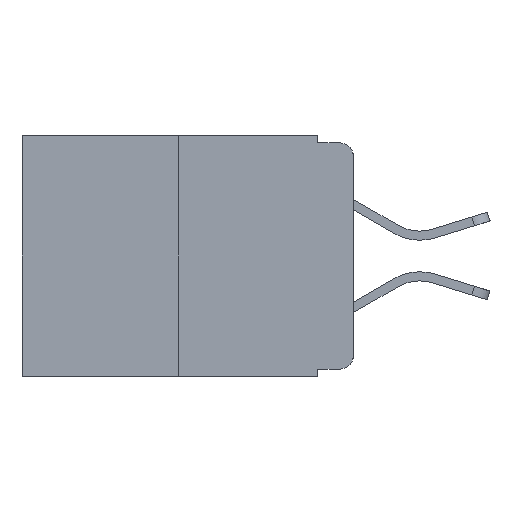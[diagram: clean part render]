
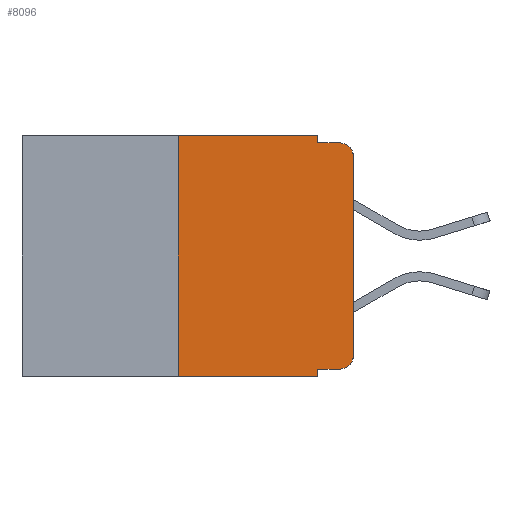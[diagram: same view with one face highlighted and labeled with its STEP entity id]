
A CAD part, left-side view. The second image highlights one B-rep face of the part: STEP entity #8096.
In plain terms, the highlighted planar face has unit normal (-1, 0, 0).
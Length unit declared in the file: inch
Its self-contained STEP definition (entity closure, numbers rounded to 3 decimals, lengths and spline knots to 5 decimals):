
#320 = VECTOR ( 'NONE', #7703, 39.37008 ) ;
#955 = VERTEX_POINT ( 'NONE', #5135 ) ;
#1524 = ORIENTED_EDGE ( 'NONE', *, *, #12093, .F. ) ;
#3200 = DIRECTION ( 'NONE',  ( 0., 0., 1. ) ) ;
#3365 = ORIENTED_EDGE ( 'NONE', *, *, #22519, .T. ) ;
#4025 = VECTOR ( 'NONE', #3200, 39.37008 ) ;
#4066 = CARTESIAN_POINT ( 'NONE',  ( 0., 0.051, 0. ) ) ;
#4126 = AXIS2_PLACEMENT_3D ( 'NONE', #4186, #17019, #6067 ) ;
#4186 = CARTESIAN_POINT ( 'NONE',  ( 0., 0.02, -0.03 ) ) ;
#4199 = ORIENTED_EDGE ( 'NONE', *, *, #20206, .F. ) ;
#4309 = EDGE_CURVE ( 'NONE', #19508, #9782, #14502, .T. ) ;
#4630 = EDGE_CURVE ( 'NONE', #11455, #955, #16774, .T. ) ;
#5101 = CARTESIAN_POINT ( 'NONE',  ( 0., 0.051, -0.343 ) ) ;
#5135 = CARTESIAN_POINT ( 'NONE',  ( 0., 0.02, -0.01 ) ) ;
#6001 = VERTEX_POINT ( 'NONE', #13910 ) ;
#6067 = DIRECTION ( 'NONE',  ( 0., 0., -1. ) ) ;
#6361 = CARTESIAN_POINT ( 'NONE',  ( 0., 0.02, -0.313 ) ) ;
#6735 = CIRCLE ( 'NONE', #9014, 0.02 ) ;
#6956 = CARTESIAN_POINT ( 'NONE',  ( 0., 0.25, 0. ) ) ;
#7387 = ORIENTED_EDGE ( 'NONE', *, *, #17792, .F. ) ;
#7703 = DIRECTION ( 'NONE',  ( 0., -1., 0. ) ) ;
#8033 = EDGE_CURVE ( 'NONE', #19508, #12342, #15763, .T. ) ;
#8096 = ADVANCED_FACE ( 'NONE', ( #14039 ), #18877, .F. ) ;
#8105 = CARTESIAN_POINT ( 'NONE',  ( 0., 0., -0.313 ) ) ;
#8190 = DIRECTION ( 'NONE',  ( 0., 0., -1. ) ) ;
#8337 = EDGE_CURVE ( 'NONE', #12122, #11455, #8857, .T. ) ;
#8559 = CARTESIAN_POINT ( 'NONE',  ( 0., 0., 0. ) ) ;
#8724 = VECTOR ( 'NONE', #10862, 39.37008 ) ;
#8857 = LINE ( 'NONE', #8559, #13734 ) ;
#9014 = AXIS2_PLACEMENT_3D ( 'NONE', #6361, #19100, #8190 ) ;
#9021 = CARTESIAN_POINT ( 'NONE',  ( 0., 0.473, 0. ) ) ;
#9195 = CARTESIAN_POINT ( 'NONE',  ( 0., 0.051, -0.01 ) ) ;
#9278 = ORIENTED_EDGE ( 'NONE', *, *, #8337, .T. ) ;
#9703 = DIRECTION ( 'NONE',  ( 1., 0., 0. ) ) ;
#9782 = VERTEX_POINT ( 'NONE', #22128 ) ;
#9829 = DIRECTION ( 'NONE',  ( 0., 0., -1. ) ) ;
#10133 = AXIS2_PLACEMENT_3D ( 'NONE', #11504, #9703, #22394 ) ;
#10418 = LINE ( 'NONE', #9021, #8724 ) ;
#10862 = DIRECTION ( 'NONE',  ( 0., -1., 0. ) ) ;
#11044 = LINE ( 'NONE', #20826, #15350 ) ;
#11102 = CARTESIAN_POINT ( 'NONE',  ( 0., 0.473, -0.343 ) ) ;
#11158 = CARTESIAN_POINT ( 'NONE',  ( 0., 0.25, -0.343 ) ) ;
#11455 = VERTEX_POINT ( 'NONE', #21836 ) ;
#11504 = CARTESIAN_POINT ( 'NONE',  ( 0., 0.473, 0. ) ) ;
#11909 = EDGE_LOOP ( 'NONE', ( #9278, #21811, #18761, #1524, #7387, #4199, #3365, #12320, #12814, #14368 ) ) ;
#12093 = EDGE_CURVE ( 'NONE', #17776, #21843, #11044, .T. ) ;
#12122 = VERTEX_POINT ( 'NONE', #8105 ) ;
#12142 = EDGE_CURVE ( 'NONE', #9782, #12122, #6735, .T. ) ;
#12320 = ORIENTED_EDGE ( 'NONE', *, *, #8033, .F. ) ;
#12342 = VERTEX_POINT ( 'NONE', #5101 ) ;
#12814 = ORIENTED_EDGE ( 'NONE', *, *, #4309, .T. ) ;
#12952 = DIRECTION ( 'NONE',  ( 0., -1., 0. ) ) ;
#13734 = VECTOR ( 'NONE', #22999, 39.37008 ) ;
#13910 = CARTESIAN_POINT ( 'NONE',  ( 0., 0.25, 0. ) ) ;
#14039 = FACE_OUTER_BOUND ( 'NONE', #11909, .T. ) ;
#14154 = DIRECTION ( 'NONE',  ( 0., -1., 0. ) ) ;
#14368 = ORIENTED_EDGE ( 'NONE', *, *, #12142, .T. ) ;
#14502 = LINE ( 'NONE', #19629, #23431 ) ;
#15035 = DIRECTION ( 'NONE',  ( 0., 0., -1. ) ) ;
#15093 = LINE ( 'NONE', #20465, #320 ) ;
#15350 = VECTOR ( 'NONE', #9829, 39.37008 ) ;
#15763 = LINE ( 'NONE', #4066, #16337 ) ;
#15911 = CARTESIAN_POINT ( 'NONE',  ( 0., 0.051, -0.333 ) ) ;
#16143 = EDGE_CURVE ( 'NONE', #21843, #955, #15093, .T. ) ;
#16337 = VECTOR ( 'NONE', #15035, 39.37008 ) ;
#16774 = CIRCLE ( 'NONE', #4126, 0.02 ) ;
#17019 = DIRECTION ( 'NONE',  ( -1., 0., 0. ) ) ;
#17776 = VERTEX_POINT ( 'NONE', #18198 ) ;
#17792 = EDGE_CURVE ( 'NONE', #6001, #17776, #10418, .T. ) ;
#18123 = LINE ( 'NONE', #6956, #4025 ) ;
#18198 = CARTESIAN_POINT ( 'NONE',  ( 0., 0.051, 0. ) ) ;
#18576 = LINE ( 'NONE', #11102, #22674 ) ;
#18761 = ORIENTED_EDGE ( 'NONE', *, *, #16143, .F. ) ;
#18877 = PLANE ( 'NONE',  #10133 ) ;
#19100 = DIRECTION ( 'NONE',  ( -1., 0., 0. ) ) ;
#19508 = VERTEX_POINT ( 'NONE', #15911 ) ;
#19629 = CARTESIAN_POINT ( 'NONE',  ( 0., 0.051, -0.333 ) ) ;
#20206 = EDGE_CURVE ( 'NONE', #21265, #6001, #18123, .T. ) ;
#20465 = CARTESIAN_POINT ( 'NONE',  ( 0., 0.051, -0.01 ) ) ;
#20826 = CARTESIAN_POINT ( 'NONE',  ( 0., 0.051, 0. ) ) ;
#21265 = VERTEX_POINT ( 'NONE', #11158 ) ;
#21811 = ORIENTED_EDGE ( 'NONE', *, *, #4630, .T. ) ;
#21836 = CARTESIAN_POINT ( 'NONE',  ( 0., 0., -0.03 ) ) ;
#21843 = VERTEX_POINT ( 'NONE', #9195 ) ;
#22128 = CARTESIAN_POINT ( 'NONE',  ( 0., 0.02, -0.333 ) ) ;
#22394 = DIRECTION ( 'NONE',  ( 0., 0., -1. ) ) ;
#22519 = EDGE_CURVE ( 'NONE', #21265, #12342, #18576, .T. ) ;
#22674 = VECTOR ( 'NONE', #12952, 39.37008 ) ;
#22999 = DIRECTION ( 'NONE',  ( 0., 0., 1. ) ) ;
#23431 = VECTOR ( 'NONE', #14154, 39.37008 ) ;
